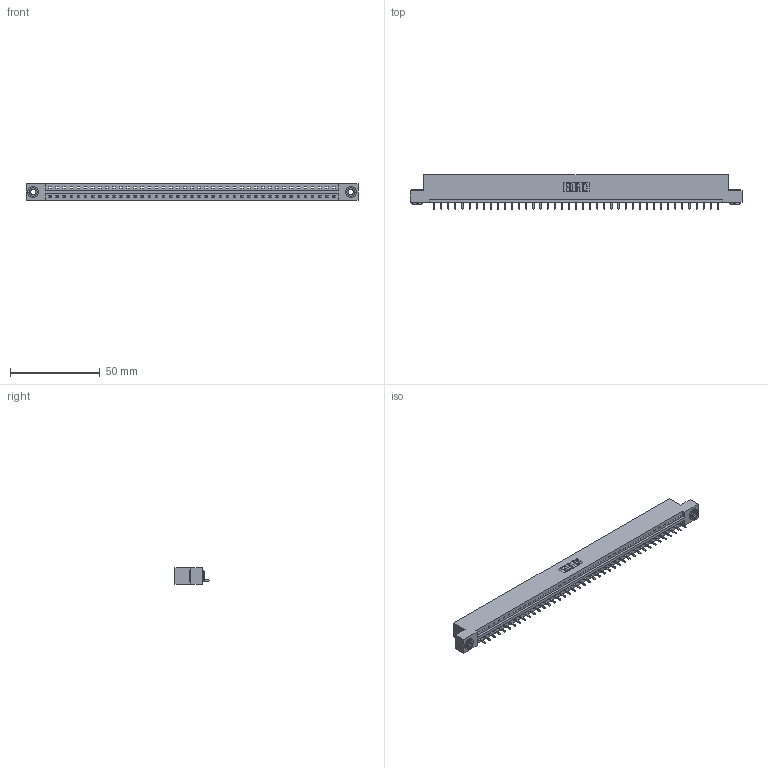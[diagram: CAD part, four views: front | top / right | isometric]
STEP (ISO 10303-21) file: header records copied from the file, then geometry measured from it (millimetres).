
FILE_DESCRIPTION (( 'STEP AP203' ), '1' );
FILE_NAME ('387-041-521-103.STEP', '2019-10-04T19:25:01', ( '' ), ( '' ), 'SwSTEP 2.0', 'SolidWorks 2016', '' );
FILE_SCHEMA (( 'CONFIG_CONTROL_DESIGN' ));
Length unit declared in the file: inch
Products named in the file (4): 345-292-001_345-293-121; 345-250-002_345-250-002-102; 387-041-521-103; 337 Part_Flush Mounting Lugs - 0.156 Dia-TH
Assembly tree (44 placements, depth 2):
  387-041-521-103
    337 Part_Flush Mounting Lugs - 0.156 Dia-TH
    345-292-001_345-293-121  x41
    345-250-002_345-250-002-102  x2
Bounding box: 185.47 x 19.06 x 9.4 mm (x, y, z)
Volume: 19166.8 mm3; surface area: 19538.7 mm2
Topology: 44 solids, 44 shells, 2694 faces, 8095 edges, 5338 vertices
Faces by surface type: plane 1966, cylinder 720, cone 8
Entity records: 31274 total; most frequent: CARTESIAN_POINT 5424, ORIENTED_EDGE 5394, DIRECTION 4601, EDGE_CURVE 2697, VECTOR 2545, LINE 2545, VERTEX_POINT 1794, AXIS2_PLACEMENT_3D 1028
